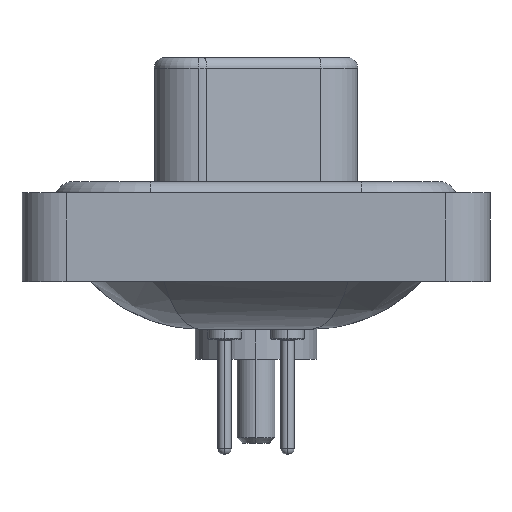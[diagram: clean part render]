
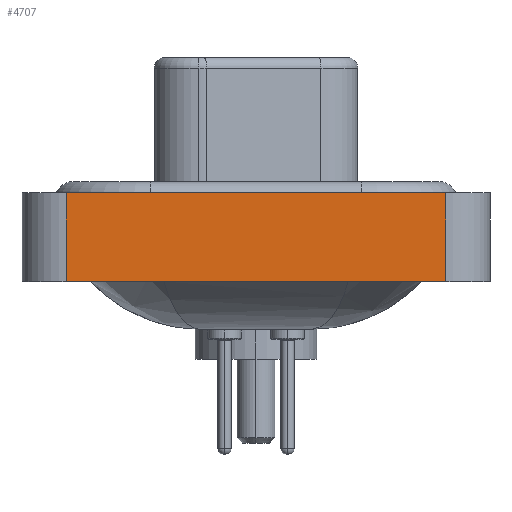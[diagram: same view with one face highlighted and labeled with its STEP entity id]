
A CAD part, left-side view. The second image highlights one B-rep face of the part: STEP entity #4707.
In plain terms, the highlighted planar face has unit normal (-1, 0, 0).
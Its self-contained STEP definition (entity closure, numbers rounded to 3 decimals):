
#588 = FACE_OUTER_BOUND ( 'NONE', #4186, .T. ) ;
#686 = DIRECTION ( 'NONE',  ( -1., 0., 0. ) ) ;
#1522 = VERTEX_POINT ( 'NONE', #3546 ) ;
#1647 = DIRECTION ( 'NONE',  ( 0., -1., 0. ) ) ;
#2177 = EDGE_CURVE ( 'NONE', #11092, #15461, #11994, .T. ) ;
#3546 = CARTESIAN_POINT ( 'NONE',  ( -7.25, -8.55, -3.6 ) ) ;
#3951 = DIRECTION ( 'NONE',  ( 0., -1., 0. ) ) ;
#4186 = EDGE_LOOP ( 'NONE', ( #10341, #4842, #10274, #8114 ) ) ;
#4613 = CARTESIAN_POINT ( 'NONE',  ( -7.25, 8.55, 0.4 ) ) ;
#4633 = CARTESIAN_POINT ( 'NONE',  ( -7.25, -8.55, -3.6 ) ) ;
#4707 = ADVANCED_FACE ( 'NONE', ( #588 ), #4722, .T. ) ;
#4722 = PLANE ( 'NONE',  #14209 ) ;
#4771 = EDGE_CURVE ( 'NONE', #11092, #1522, #11243, .T. ) ;
#4842 = ORIENTED_EDGE ( 'NONE', *, *, #11692, .F. ) ;
#7407 = CARTESIAN_POINT ( 'NONE',  ( -7.25, 8.55, -3.6 ) ) ;
#8030 = VERTEX_POINT ( 'NONE', #12697 ) ;
#8114 = ORIENTED_EDGE ( 'NONE', *, *, #4771, .T. ) ;
#9173 = VECTOR ( 'NONE', #3951, 1000. ) ;
#9504 = LINE ( 'NONE', #16236, #9173 ) ;
#9986 = DIRECTION ( 'NONE',  ( 0., 0., 1. ) ) ;
#10094 = CARTESIAN_POINT ( 'NONE',  ( -7.25, -8.55, -3.6 ) ) ;
#10274 = ORIENTED_EDGE ( 'NONE', *, *, #2177, .F. ) ;
#10341 = ORIENTED_EDGE ( 'NONE', *, *, #12526, .T. ) ;
#10486 = CARTESIAN_POINT ( 'NONE',  ( -7.25, 8.55, -3.6 ) ) ;
#11092 = VERTEX_POINT ( 'NONE', #7407 ) ;
#11243 = LINE ( 'NONE', #16557, #15917 ) ;
#11692 = EDGE_CURVE ( 'NONE', #15461, #8030, #9504, .T. ) ;
#11994 = LINE ( 'NONE', #10486, #16874 ) ;
#12526 = EDGE_CURVE ( 'NONE', #1522, #8030, #12850, .T. ) ;
#12697 = CARTESIAN_POINT ( 'NONE',  ( -7.25, -8.55, 0.4 ) ) ;
#12850 = LINE ( 'NONE', #10094, #16773 ) ;
#13254 = DIRECTION ( 'NONE',  ( 0., 0., 1. ) ) ;
#14209 = AXIS2_PLACEMENT_3D ( 'NONE', #4633, #686, #9986 ) ;
#15461 = VERTEX_POINT ( 'NONE', #4613 ) ;
#15917 = VECTOR ( 'NONE', #1647, 1000. ) ;
#16236 = CARTESIAN_POINT ( 'NONE',  ( -7.25, -8.55, 0.4 ) ) ;
#16557 = CARTESIAN_POINT ( 'NONE',  ( -7.25, -8.55, -3.6 ) ) ;
#16734 = DIRECTION ( 'NONE',  ( 0., 0., 1. ) ) ;
#16773 = VECTOR ( 'NONE', #16734, 1000. ) ;
#16874 = VECTOR ( 'NONE', #13254, 1000. ) ;
